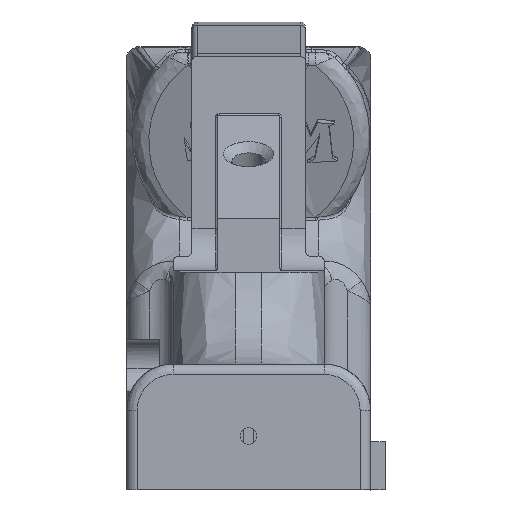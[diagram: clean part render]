
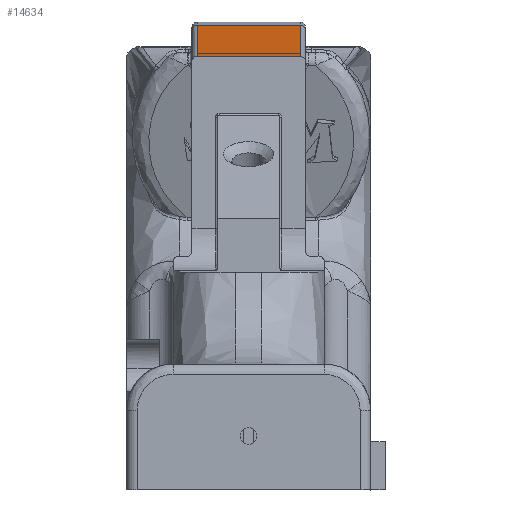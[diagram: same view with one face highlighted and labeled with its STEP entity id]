
A CAD part, left-side view. The second image highlights one B-rep face of the part: STEP entity #14634.
In plain terms, the highlighted face is planar.
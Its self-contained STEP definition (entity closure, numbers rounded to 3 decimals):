
#511 = CARTESIAN_POINT ( 'NONE',  ( -131.218, -60.89, -7.55 ) ) ;
#663 = VECTOR ( 'NONE', #13956, 1000. ) ;
#1174 = ORIENTED_EDGE ( 'NONE', *, *, #8685, .T. ) ;
#1542 = LINE ( 'NONE', #8290, #11957 ) ;
#1561 = ORIENTED_EDGE ( 'NONE', *, *, #12143, .T. ) ;
#1882 = EDGE_CURVE ( 'NONE', #15197, #13496, #15857, .T. ) ;
#2124 = DIRECTION ( 'NONE',  ( 0., 0., 1. ) ) ;
#2154 = CARTESIAN_POINT ( 'NONE',  ( -131.112, -60.913, 7.394 ) ) ;
#2306 = VECTOR ( 'NONE', #2124, 1000. ) ;
#2848 = ORIENTED_EDGE ( 'NONE', *, *, #19830, .T. ) ;
#3105 = DIRECTION ( 'NONE',  ( 0., 0., -1. ) ) ;
#3160 = ORIENTED_EDGE ( 'NONE', *, *, #21193, .F. ) ;
#3164 = CARTESIAN_POINT ( 'NONE',  ( -133.166, -60.454, -7.855 ) ) ;
#3937 = CARTESIAN_POINT ( 'NONE',  ( -131.112, -60.913, 7.394 ) ) ;
#4077 = EDGE_CURVE ( 'NONE', #13516, #14530, #1542, .T. ) ;
#4350 = LINE ( 'NONE', #5502, #8683 ) ;
#4435 = CARTESIAN_POINT ( 'NONE',  ( -112., -65.186, 7.855 ) ) ;
#4826 = VECTOR ( 'NONE', #3105, 1000. ) ;
#5502 = CARTESIAN_POINT ( 'NONE',  ( -133.166, -60.454, 67.339 ) ) ;
#5614 = VERTEX_POINT ( 'NONE', #16222 ) ;
#6069 = CARTESIAN_POINT ( 'NONE',  ( -126.111, -62.031, 7.855 ) ) ;
#6138 = FACE_OUTER_BOUND ( 'NONE', #13937, .T. ) ;
#6429 = DIRECTION ( 'NONE',  ( -0.218, -0.976, 0. ) ) ;
#6582 = ORIENTED_EDGE ( 'NONE', *, *, #1882, .T. ) ;
#6943 = VERTEX_POINT ( 'NONE', #13170 ) ;
#8290 = CARTESIAN_POINT ( 'NONE',  ( -133.166, -60.454, -7.855 ) ) ;
#8683 = VECTOR ( 'NONE', #10688, 1000. ) ;
#8685 = EDGE_CURVE ( 'NONE', #6943, #11094, #20900, .T. ) ;
#8865 = EDGE_CURVE ( 'NONE', #11094, #15197, #13113, .T. ) ;
#9038 = CARTESIAN_POINT ( 'NONE',  ( -131.439, -60.84, 7.854 ) ) ;
#9154 = CARTESIAN_POINT ( 'NONE',  ( -131.439, -60.84, -7.854 ) ) ;
#9779 = CARTESIAN_POINT ( 'NONE',  ( -119.056, -63.608, 7.855 ) ) ;
#9972 = CARTESIAN_POINT ( 'NONE',  ( -133.166, -60.454, 67.339 ) ) ;
#10688 = DIRECTION ( 'NONE',  ( 0., 0., -1. ) ) ;
#10961 = ORIENTED_EDGE ( 'NONE', *, *, #20384, .T. ) ;
#11094 = VERTEX_POINT ( 'NONE', #2154 ) ;
#11366 = CARTESIAN_POINT ( 'NONE',  ( -131.112, -60.913, -7.394 ) ) ;
#11688 = DIRECTION ( 'NONE',  ( 0.976, -0.218, 0. ) ) ;
#11957 = VECTOR ( 'NONE', #16981, 1000. ) ;
#12143 = EDGE_CURVE ( 'NONE', #5614, #15129, #17711, .T. ) ;
#12660 = LINE ( 'NONE', #19056, #663 ) ;
#13053 = CARTESIAN_POINT ( 'NONE',  ( -133.166, -60.454, 7.855 ) ) ;
#13089 = CARTESIAN_POINT ( 'NONE',  ( -131.439, -60.84, -7.854 ) ) ;
#13113 = LINE ( 'NONE', #21713, #4826 ) ;
#13170 = CARTESIAN_POINT ( 'NONE',  ( -131.439, -60.84, 7.854 ) ) ;
#13496 = VERTEX_POINT ( 'NONE', #13089 ) ;
#13516 = VERTEX_POINT ( 'NONE', #3164 ) ;
#13718 = AXIS2_PLACEMENT_3D ( 'NONE', #9972, #6429, #11688 ) ;
#13792 = LINE ( 'NONE', #15651, #2306 ) ;
#13937 = EDGE_LOOP ( 'NONE', ( #10961, #16004, #3160, #1561 ) ) ;
#13938 = FACE_BOUND ( 'NONE', #17350, .T. ) ;
#13956 = DIRECTION ( 'NONE',  ( 0., 0., -1. ) ) ;
#14398 = ORIENTED_EDGE ( 'NONE', *, *, #8865, .T. ) ;
#14530 = VERTEX_POINT ( 'NONE', #19604 ) ;
#14634 = ADVANCED_FACE ( 'NONE', ( #13938, #6138 ), #18331, .T. ) ;
#15129 = VERTEX_POINT ( 'NONE', #13053 ) ;
#15197 = VERTEX_POINT ( 'NONE', #11366 ) ;
#15651 = CARTESIAN_POINT ( 'NONE',  ( -131.439, -60.84, 67.339 ) ) ;
#15857 = B_SPLINE_CURVE_WITH_KNOTS ( 'NONE', 3,
 ( #17884, #511, #17670, #9154 ),
 .UNSPECIFIED., .F., .F.,
 ( 4, 4 ),
 ( 0., 1. ),
 .UNSPECIFIED. ) ;
#16004 = ORIENTED_EDGE ( 'NONE', *, *, #4077, .T. ) ;
#16222 = CARTESIAN_POINT ( 'NONE',  ( -112., -65.186, 7.855 ) ) ;
#16981 = DIRECTION ( 'NONE',  ( 0.976, -0.218, 0. ) ) ;
#17350 = EDGE_LOOP ( 'NONE', ( #14398, #6582, #2848, #1174 ) ) ;
#17670 = CARTESIAN_POINT ( 'NONE',  ( -131.327, -60.865, -7.703 ) ) ;
#17711 = B_SPLINE_CURVE_WITH_KNOTS ( 'NONE', 3,
 ( #4435, #9779, #6069, #21721 ),
 .UNSPECIFIED., .F., .F.,
 ( 4, 4 ),
 ( 0., 1. ),
 .UNSPECIFIED. ) ;
#17838 = CARTESIAN_POINT ( 'NONE',  ( -131.327, -60.865, 7.703 ) ) ;
#17884 = CARTESIAN_POINT ( 'NONE',  ( -131.112, -60.913, -7.394 ) ) ;
#18331 = PLANE ( 'NONE',  #13718 ) ;
#19056 = CARTESIAN_POINT ( 'NONE',  ( -112., -65.186, 67.339 ) ) ;
#19424 = CARTESIAN_POINT ( 'NONE',  ( -131.218, -60.89, 7.55 ) ) ;
#19604 = CARTESIAN_POINT ( 'NONE',  ( -112., -65.186, -7.855 ) ) ;
#19830 = EDGE_CURVE ( 'NONE', #13496, #6943, #13792, .T. ) ;
#20384 = EDGE_CURVE ( 'NONE', #15129, #13516, #4350, .T. ) ;
#20900 = B_SPLINE_CURVE_WITH_KNOTS ( 'NONE', 3,
 ( #9038, #17838, #19424, #3937 ),
 .UNSPECIFIED., .F., .F.,
 ( 4, 4 ),
 ( 0., 1. ),
 .UNSPECIFIED. ) ;
#21193 = EDGE_CURVE ( 'NONE', #5614, #14530, #12660, .T. ) ;
#21713 = CARTESIAN_POINT ( 'NONE',  ( -131.112, -60.913, 67.339 ) ) ;
#21721 = CARTESIAN_POINT ( 'NONE',  ( -133.166, -60.454, 7.855 ) ) ;
